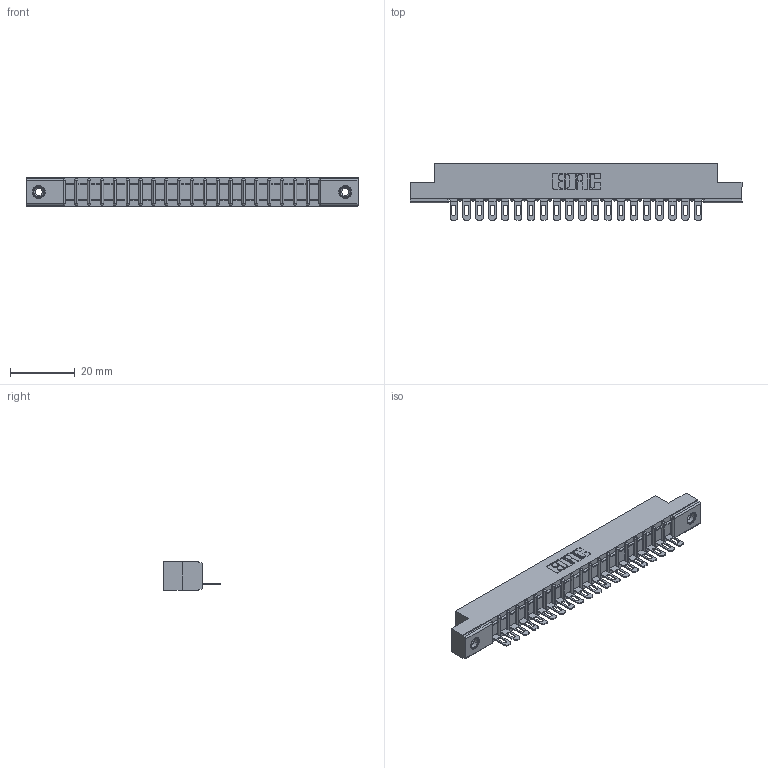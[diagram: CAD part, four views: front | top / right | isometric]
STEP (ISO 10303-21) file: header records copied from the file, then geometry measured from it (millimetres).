
FILE_DESCRIPTION (( 'STEP AP203' ), '1' );
FILE_NAME ('357-020-501-108.STEP', '2018-08-08T07:53:13', ( '' ), ( '' ), 'SwSTEP 2.0', 'SolidWorks 2016', '' );
FILE_SCHEMA (( 'CONFIG_CONTROL_DESIGN' ));
Length unit declared in the file: inch
Products named in the file (4): 307 Part_.156 Dia Mounting Holes; 307-290-002_501; 345-250-001_345-250-003-102; 357-020-501-108
Assembly tree (23 placements, depth 2):
  357-020-501-108
    307 Part_.156 Dia Mounting Holes
    307-290-002_501  x20
    345-250-001_345-250-003-102  x2
Bounding box: 102.26 x 17.42 x 8.71 mm (x, y, z)
Volume: 6760.9 mm3; surface area: 12339.1 mm2
Topology: 23 solids, 23 shells, 1719 faces, 5219 edges, 3414 vertices
Faces by surface type: plane 982, cylinder 679, sphere 42, cone 12, torus 4
Entity records: 21837 total; most frequent: CARTESIAN_POINT 3659, ORIENTED_EDGE 3642, DIRECTION 3579, EDGE_CURVE 1821, VECTOR 1379, LINE 1379, VERTEX_POINT 1180, AXIS2_PLACEMENT_3D 1100
